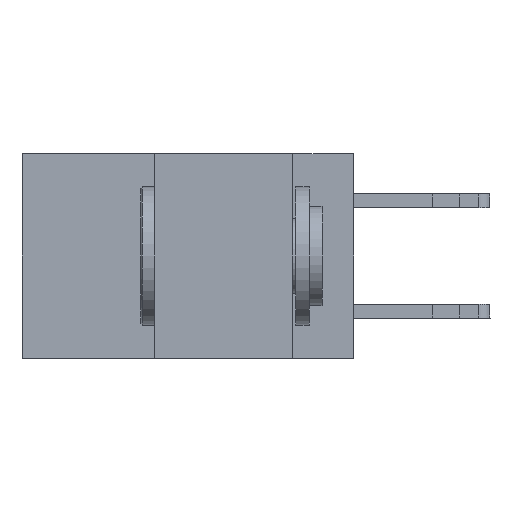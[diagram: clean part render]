
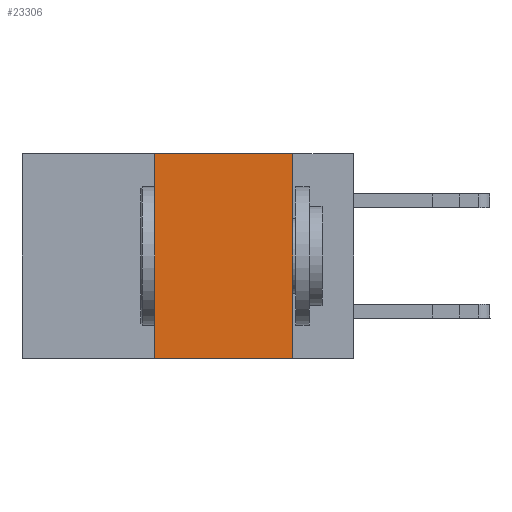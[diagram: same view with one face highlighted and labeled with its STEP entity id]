
A CAD part, left-side view. The second image highlights one B-rep face of the part: STEP entity #23306.
In plain terms, the highlighted planar face has unit normal (-1, 0, 0).
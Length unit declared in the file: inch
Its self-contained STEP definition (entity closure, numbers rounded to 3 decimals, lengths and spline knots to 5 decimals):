
#247 = LINE ( 'NONE', #4367, #14449 ) ;
#2228 = VERTEX_POINT ( 'NONE', #20581 ) ;
#4367 = CARTESIAN_POINT ( 'NONE',  ( 0., 0.11, 0. ) ) ;
#4852 = PLANE ( 'NONE',  #23388 ) ;
#4932 = DIRECTION ( 'NONE',  ( 1., 0., 0. ) ) ;
#6403 = ORIENTED_EDGE ( 'NONE', *, *, #18324, .F. ) ;
#6855 = VERTEX_POINT ( 'NONE', #22028 ) ;
#7285 = EDGE_CURVE ( 'NONE', #2228, #12028, #18593, .T. ) ;
#7462 = EDGE_LOOP ( 'NONE', ( #6403, #21677, #13729, #23372 ) ) ;
#7769 = DIRECTION ( 'NONE',  ( 0., 0., 1. ) ) ;
#8013 = DIRECTION ( 'NONE',  ( 0., 0., -1. ) ) ;
#8211 = CARTESIAN_POINT ( 'NONE',  ( 0., 0.6, -0.37 ) ) ;
#8353 = EDGE_CURVE ( 'NONE', #6855, #22788, #9335, .T. ) ;
#8552 = DIRECTION ( 'NONE',  ( 0., -1., 0. ) ) ;
#9335 = LINE ( 'NONE', #8211, #18578 ) ;
#10154 = DIRECTION ( 'NONE',  ( 0., -1., 0. ) ) ;
#11723 = VECTOR ( 'NONE', #7769, 39.37008 ) ;
#12028 = VERTEX_POINT ( 'NONE', #16990 ) ;
#12681 = CARTESIAN_POINT ( 'NONE',  ( 0., 0.11, -0.37 ) ) ;
#13169 = VECTOR ( 'NONE', #8552, 39.37008 ) ;
#13427 = EDGE_CURVE ( 'NONE', #6855, #2228, #16633, .T. ) ;
#13729 = ORIENTED_EDGE ( 'NONE', *, *, #13427, .F. ) ;
#14449 = VECTOR ( 'NONE', #8013, 39.37008 ) ;
#16034 = CARTESIAN_POINT ( 'NONE',  ( 0., 0.6, 0. ) ) ;
#16633 = LINE ( 'NONE', #17164, #11723 ) ;
#16990 = CARTESIAN_POINT ( 'NONE',  ( 0., 0.11, 0. ) ) ;
#17164 = CARTESIAN_POINT ( 'NONE',  ( 0., 0.36, 0. ) ) ;
#17740 = CARTESIAN_POINT ( 'NONE',  ( 0., 0.6, 0. ) ) ;
#17868 = DIRECTION ( 'NONE',  ( 0., 0., -1. ) ) ;
#18324 = EDGE_CURVE ( 'NONE', #12028, #22788, #247, .T. ) ;
#18578 = VECTOR ( 'NONE', #10154, 39.37008 ) ;
#18593 = LINE ( 'NONE', #17740, #13169 ) ;
#19048 = FACE_OUTER_BOUND ( 'NONE', #7462, .T. ) ;
#20581 = CARTESIAN_POINT ( 'NONE',  ( 0., 0.36, 0. ) ) ;
#21677 = ORIENTED_EDGE ( 'NONE', *, *, #7285, .F. ) ;
#22028 = CARTESIAN_POINT ( 'NONE',  ( 0., 0.36, -0.37 ) ) ;
#22788 = VERTEX_POINT ( 'NONE', #12681 ) ;
#23306 = ADVANCED_FACE ( 'NONE', ( #19048 ), #4852, .F. ) ;
#23372 = ORIENTED_EDGE ( 'NONE', *, *, #8353, .T. ) ;
#23388 = AXIS2_PLACEMENT_3D ( 'NONE', #16034, #4932, #17868 ) ;
